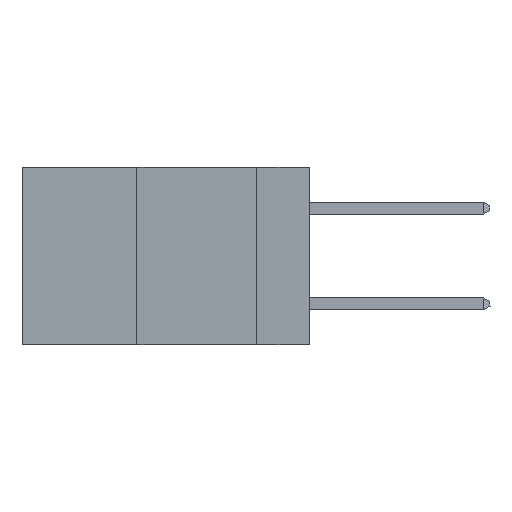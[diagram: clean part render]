
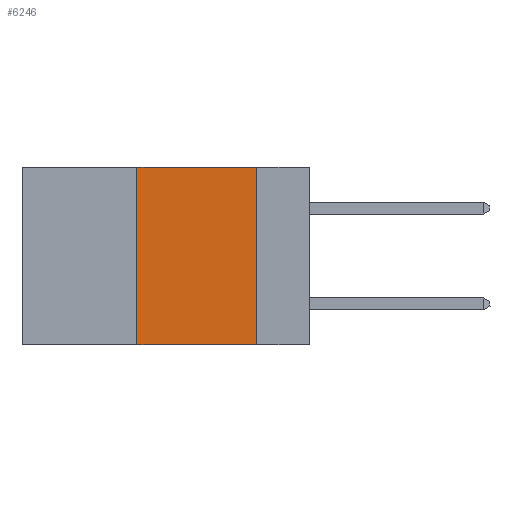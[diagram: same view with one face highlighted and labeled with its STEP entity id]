
A CAD part, left-side view. The second image highlights one B-rep face of the part: STEP entity #6246.
In plain terms, the highlighted planar face has unit normal (-1, 0, 0).
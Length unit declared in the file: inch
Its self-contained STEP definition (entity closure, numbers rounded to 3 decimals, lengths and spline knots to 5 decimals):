
#104 = ORIENTED_EDGE ( 'NONE', *, *, #13337, .F. ) ;
#229 = LINE ( 'NONE', #10990, #15585 ) ;
#811 = VERTEX_POINT ( 'NONE', #4653 ) ;
#976 = LINE ( 'NONE', #10559, #14200 ) ;
#1160 = CARTESIAN_POINT ( 'NONE',  ( 0., 0.36, -0.37 ) ) ;
#1301 = CARTESIAN_POINT ( 'NONE',  ( 0., 0.6, 0. ) ) ;
#1392 = FACE_OUTER_BOUND ( 'NONE', #5746, .T. ) ;
#2356 = EDGE_CURVE ( 'NONE', #811, #13894, #5235, .T. ) ;
#2697 = PLANE ( 'NONE',  #6005 ) ;
#2747 = CARTESIAN_POINT ( 'NONE',  ( 0., 0.6, 0. ) ) ;
#3484 = CARTESIAN_POINT ( 'NONE',  ( 0., 0.11, 0. ) ) ;
#3538 = DIRECTION ( 'NONE',  ( 0., 0., -1. ) ) ;
#4653 = CARTESIAN_POINT ( 'NONE',  ( 0., 0.36, 0. ) ) ;
#5235 = LINE ( 'NONE', #1301, #7191 ) ;
#5746 = EDGE_LOOP ( 'NONE', ( #104, #10656, #13672, #15057 ) ) ;
#6005 = AXIS2_PLACEMENT_3D ( 'NONE', #2747, #10534, #3538 ) ;
#6246 = ADVANCED_FACE ( 'NONE', ( #1392 ), #2697, .F. ) ;
#6256 = CARTESIAN_POINT ( 'NONE',  ( 0., 0.11, 0. ) ) ;
#6770 = DIRECTION ( 'NONE',  ( 0., -1., 0. ) ) ;
#7068 = VERTEX_POINT ( 'NONE', #10423 ) ;
#7172 = DIRECTION ( 'NONE',  ( 0., 0., -1. ) ) ;
#7191 = VECTOR ( 'NONE', #15001, 39.37008 ) ;
#7213 = DIRECTION ( 'NONE',  ( 0., 0., 1. ) ) ;
#8181 = LINE ( 'NONE', #3484, #14386 ) ;
#10423 = CARTESIAN_POINT ( 'NONE',  ( 0., 0.11, -0.37 ) ) ;
#10534 = DIRECTION ( 'NONE',  ( 1., 0., 0. ) ) ;
#10559 = CARTESIAN_POINT ( 'NONE',  ( 0., 0.6, -0.37 ) ) ;
#10656 = ORIENTED_EDGE ( 'NONE', *, *, #2356, .F. ) ;
#10990 = CARTESIAN_POINT ( 'NONE',  ( 0., 0.36, 0. ) ) ;
#12642 = EDGE_CURVE ( 'NONE', #13126, #811, #229, .T. ) ;
#12811 = EDGE_CURVE ( 'NONE', #13126, #7068, #976, .T. ) ;
#13126 = VERTEX_POINT ( 'NONE', #1160 ) ;
#13337 = EDGE_CURVE ( 'NONE', #13894, #7068, #8181, .T. ) ;
#13672 = ORIENTED_EDGE ( 'NONE', *, *, #12642, .F. ) ;
#13894 = VERTEX_POINT ( 'NONE', #6256 ) ;
#14200 = VECTOR ( 'NONE', #6770, 39.37008 ) ;
#14386 = VECTOR ( 'NONE', #7172, 39.37008 ) ;
#15001 = DIRECTION ( 'NONE',  ( 0., -1., 0. ) ) ;
#15057 = ORIENTED_EDGE ( 'NONE', *, *, #12811, .T. ) ;
#15585 = VECTOR ( 'NONE', #7213, 39.37008 ) ;
